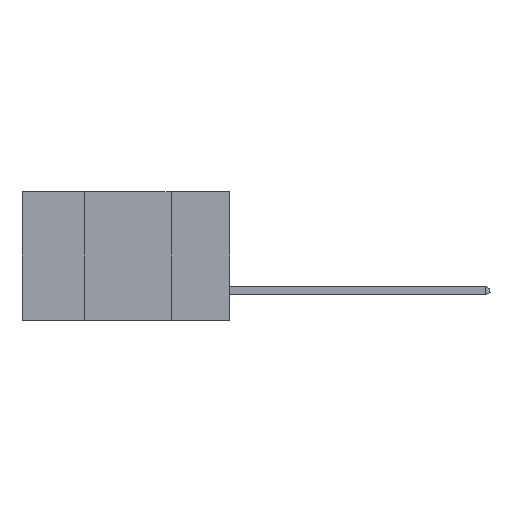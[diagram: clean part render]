
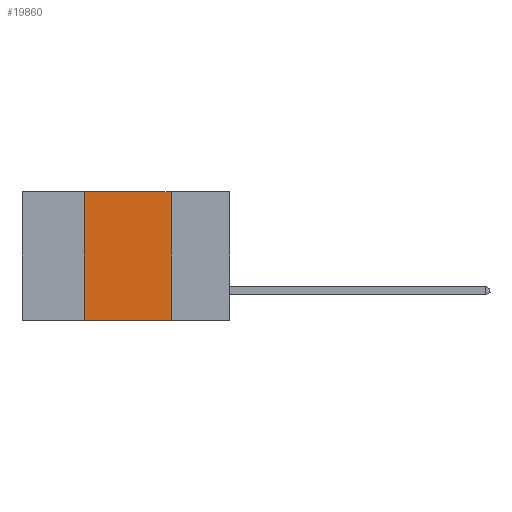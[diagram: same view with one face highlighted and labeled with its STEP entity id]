
A CAD part, left-side view. The second image highlights one B-rep face of the part: STEP entity #19860.
In plain terms, the highlighted planar face has unit normal (-1, 0, 0).
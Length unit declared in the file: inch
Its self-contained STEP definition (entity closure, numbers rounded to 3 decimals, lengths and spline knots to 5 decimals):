
#222 = DIRECTION ( 'NONE',  ( 0., 0., 1. ) ) ;
#1036 = CARTESIAN_POINT ( 'NONE',  ( 0., 0.42, 0. ) ) ;
#3547 = LINE ( 'NONE', #16357, #13373 ) ;
#3584 = CARTESIAN_POINT ( 'NONE',  ( 0., 0.42, -0.37 ) ) ;
#7607 = VERTEX_POINT ( 'NONE', #1036 ) ;
#7727 = PLANE ( 'NONE',  #29309 ) ;
#9551 = ORIENTED_EDGE ( 'NONE', *, *, #25320, .F. ) ;
#10360 = VECTOR ( 'NONE', #23019, 39.37008 ) ;
#11579 = VERTEX_POINT ( 'NONE', #3584 ) ;
#12260 = FACE_OUTER_BOUND ( 'NONE', #20179, .T. ) ;
#13029 = VERTEX_POINT ( 'NONE', #18474 ) ;
#13373 = VECTOR ( 'NONE', #23801, 39.37008 ) ;
#14886 = LINE ( 'NONE', #26429, #19439 ) ;
#15361 = DIRECTION ( 'NONE',  ( 1., 0., 0. ) ) ;
#15587 = ORIENTED_EDGE ( 'NONE', *, *, #29418, .T. ) ;
#15775 = CARTESIAN_POINT ( 'NONE',  ( 0., 0.6, -0.37 ) ) ;
#16357 = CARTESIAN_POINT ( 'NONE',  ( 0., 0.17, 0. ) ) ;
#17456 = CARTESIAN_POINT ( 'NONE',  ( 0., 0.6, 0. ) ) ;
#17554 = LINE ( 'NONE', #15775, #10360 ) ;
#17770 = ORIENTED_EDGE ( 'NONE', *, *, #20427, .F. ) ;
#18408 = CARTESIAN_POINT ( 'NONE',  ( 0., 0.17, 0. ) ) ;
#18474 = CARTESIAN_POINT ( 'NONE',  ( 0., 0.17, -0.37 ) ) ;
#18713 = LINE ( 'NONE', #19161, #29749 ) ;
#19095 = DIRECTION ( 'NONE',  ( 0., -1., 0. ) ) ;
#19161 = CARTESIAN_POINT ( 'NONE',  ( 0., 0.42, 0. ) ) ;
#19439 = VECTOR ( 'NONE', #19095, 39.37008 ) ;
#19860 = ADVANCED_FACE ( 'NONE', ( #12260 ), #7727, .F. ) ;
#20179 = EDGE_LOOP ( 'NONE', ( #17770, #9551, #26714, #15587 ) ) ;
#20427 = EDGE_CURVE ( 'NONE', #27620, #13029, #3547, .T. ) ;
#23019 = DIRECTION ( 'NONE',  ( 0., -1., 0. ) ) ;
#23801 = DIRECTION ( 'NONE',  ( 0., 0., -1. ) ) ;
#24797 = DIRECTION ( 'NONE',  ( 0., 0., -1. ) ) ;
#25320 = EDGE_CURVE ( 'NONE', #7607, #27620, #14886, .T. ) ;
#26429 = CARTESIAN_POINT ( 'NONE',  ( 0., 0.6, 0. ) ) ;
#26714 = ORIENTED_EDGE ( 'NONE', *, *, #29153, .F. ) ;
#27620 = VERTEX_POINT ( 'NONE', #18408 ) ;
#29153 = EDGE_CURVE ( 'NONE', #11579, #7607, #18713, .T. ) ;
#29309 = AXIS2_PLACEMENT_3D ( 'NONE', #17456, #15361, #24797 ) ;
#29418 = EDGE_CURVE ( 'NONE', #11579, #13029, #17554, .T. ) ;
#29749 = VECTOR ( 'NONE', #222, 39.37008 ) ;
